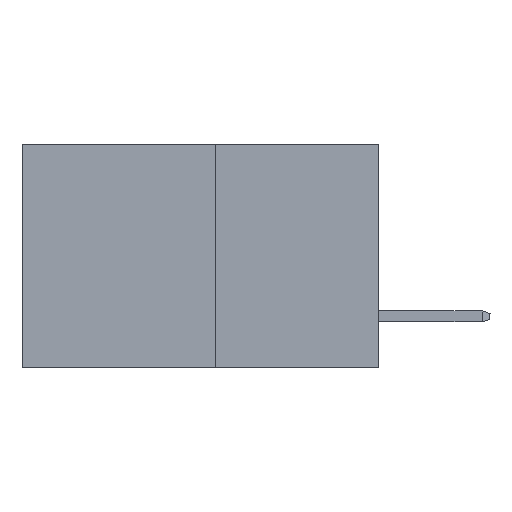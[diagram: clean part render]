
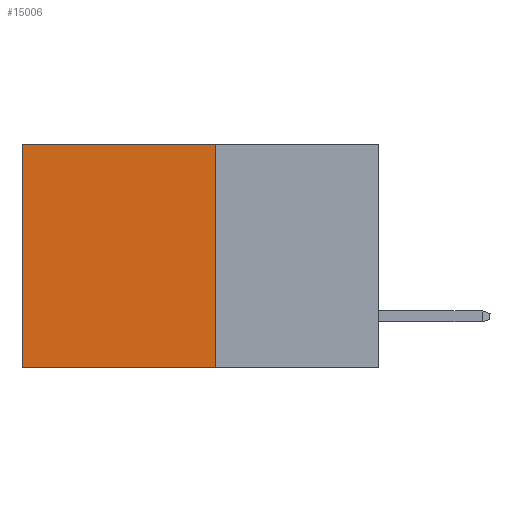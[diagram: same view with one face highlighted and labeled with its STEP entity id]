
A CAD part, left-side view. The second image highlights one B-rep face of the part: STEP entity #15006.
In plain terms, the highlighted planar face has unit normal (-1, 0, 0).
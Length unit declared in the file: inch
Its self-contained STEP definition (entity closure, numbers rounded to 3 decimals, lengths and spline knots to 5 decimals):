
#1009 = EDGE_LOOP ( 'NONE', ( #20625, #8629, #20735, #21558 ) ) ;
#3463 = VERTEX_POINT ( 'NONE', #20536 ) ;
#3950 = FACE_OUTER_BOUND ( 'NONE', #1009, .T. ) ;
#5449 = CARTESIAN_POINT ( 'NONE',  ( 0.277, 0.27, -0.37 ) ) ;
#5530 = VECTOR ( 'NONE', #9412, 39.37008 ) ;
#5762 = PLANE ( 'NONE',  #20620 ) ;
#6230 = DIRECTION ( 'NONE',  ( 0., 0., -1. ) ) ;
#6298 = VERTEX_POINT ( 'NONE', #23354 ) ;
#6648 = CARTESIAN_POINT ( 'NONE',  ( 0.277, 0.27, 0. ) ) ;
#8050 = DIRECTION ( 'NONE',  ( 0., 1., 0. ) ) ;
#8130 = LINE ( 'NONE', #24248, #27791 ) ;
#8629 = ORIENTED_EDGE ( 'NONE', *, *, #21012, .F. ) ;
#9412 = DIRECTION ( 'NONE',  ( 0., 1., 0. ) ) ;
#11021 = DIRECTION ( 'NONE',  ( 1., 0., 0. ) ) ;
#12068 = EDGE_CURVE ( 'NONE', #3463, #18879, #8130, .T. ) ;
#13291 = VECTOR ( 'NONE', #8050, 39.37008 ) ;
#14203 = EDGE_CURVE ( 'NONE', #6298, #29332, #29635, .T. ) ;
#15006 = ADVANCED_FACE ( 'NONE', ( #3950 ), #5762, .F. ) ;
#18879 = VERTEX_POINT ( 'NONE', #23988 ) ;
#19322 = LINE ( 'NONE', #6648, #5530 ) ;
#20536 = CARTESIAN_POINT ( 'NONE',  ( 0.277, 0.27, 0. ) ) ;
#20620 = AXIS2_PLACEMENT_3D ( 'NONE', #26320, #11021, #28852 ) ;
#20625 = ORIENTED_EDGE ( 'NONE', *, *, #14203, .T. ) ;
#20735 = ORIENTED_EDGE ( 'NONE', *, *, #12068, .F. ) ;
#21012 = EDGE_CURVE ( 'NONE', #18879, #29332, #26859, .T. ) ;
#21558 = ORIENTED_EDGE ( 'NONE', *, *, #30808, .T. ) ;
#21629 = CARTESIAN_POINT ( 'NONE',  ( 0.277, 0.59, -0.37 ) ) ;
#23137 = CARTESIAN_POINT ( 'NONE',  ( 0.277, 0.59, -0.37 ) ) ;
#23354 = CARTESIAN_POINT ( 'NONE',  ( 0.277, 0.59, 0. ) ) ;
#23988 = CARTESIAN_POINT ( 'NONE',  ( 0.277, 0.27, -0.37 ) ) ;
#24248 = CARTESIAN_POINT ( 'NONE',  ( 0.277, 0.27, -0.37 ) ) ;
#25820 = DIRECTION ( 'NONE',  ( 0., 0., -1. ) ) ;
#26320 = CARTESIAN_POINT ( 'NONE',  ( 0.277, 0.27, -0.37 ) ) ;
#26859 = LINE ( 'NONE', #5449, #13291 ) ;
#27791 = VECTOR ( 'NONE', #6230, 39.37008 ) ;
#28852 = DIRECTION ( 'NONE',  ( 0., 0., -1. ) ) ;
#28853 = VECTOR ( 'NONE', #25820, 39.37008 ) ;
#29332 = VERTEX_POINT ( 'NONE', #21629 ) ;
#29635 = LINE ( 'NONE', #23137, #28853 ) ;
#30808 = EDGE_CURVE ( 'NONE', #3463, #6298, #19322, .T. ) ;
